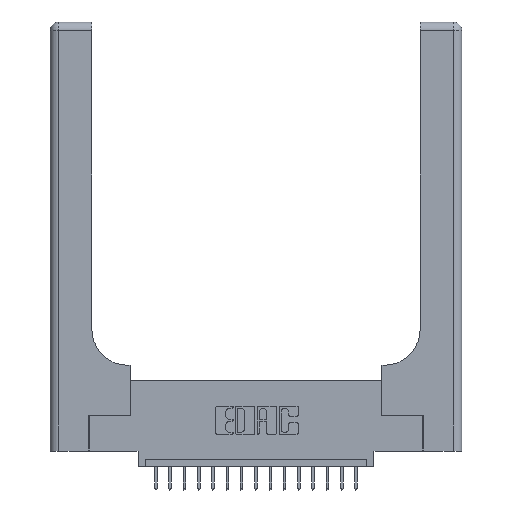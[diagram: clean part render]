
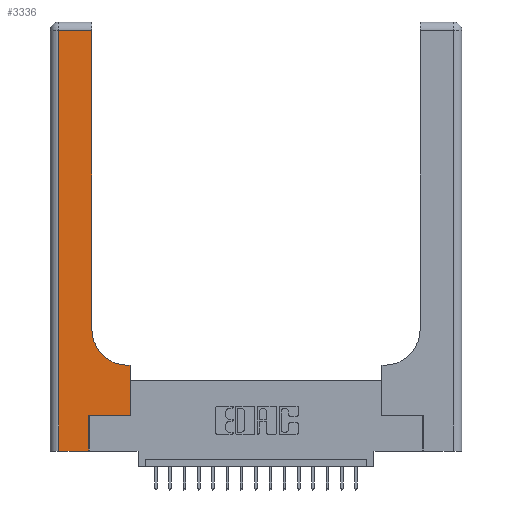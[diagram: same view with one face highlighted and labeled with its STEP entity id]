
A CAD part, top view. The second image highlights one B-rep face of the part: STEP entity #3336.
In plain terms, the highlighted planar face has unit normal (0, 0, 1).
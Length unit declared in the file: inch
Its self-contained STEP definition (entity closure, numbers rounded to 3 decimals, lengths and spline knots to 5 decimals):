
#299 = CARTESIAN_POINT ( 'NONE',  ( 0.5585, 0.6, 0.37 ) ) ;
#445 = DIRECTION ( 'NONE',  ( 1., 0., 0. ) ) ;
#703 = DIRECTION ( 'NONE',  ( 0., 1., 0. ) ) ;
#721 = LINE ( 'NONE', #16272, #4425 ) ;
#781 = ORIENTED_EDGE ( 'NONE', *, *, #13419, .T. ) ;
#2010 = CARTESIAN_POINT ( 'NONE',  ( 0.269, 0., 0.37 ) ) ;
#2020 = ORIENTED_EDGE ( 'NONE', *, *, #5002, .T. ) ;
#2302 = VERTEX_POINT ( 'NONE', #16727 ) ;
#2441 = CIRCLE ( 'NONE', #20282, 0.25 ) ;
#2905 = FACE_OUTER_BOUND ( 'NONE', #6049, .T. ) ;
#2906 = CARTESIAN_POINT ( 'NONE',  ( 0.2915, 0.6, 0.37 ) ) ;
#3103 = VECTOR ( 'NONE', #10601, 39.37008 ) ;
#3206 = VECTOR ( 'NONE', #17125, 39.37008 ) ;
#3258 = CARTESIAN_POINT ( 'NONE',  ( 0.06, 0., 0.37 ) ) ;
#3336 = ADVANCED_FACE ( 'NONE', ( #2905 ), #9201, .F. ) ;
#4198 = VERTEX_POINT ( 'NONE', #6882 ) ;
#4246 = LINE ( 'NONE', #16491, #17465 ) ;
#4425 = VECTOR ( 'NONE', #445, 39.37008 ) ;
#4515 = VECTOR ( 'NONE', #7866, 39.37008 ) ;
#4678 = AXIS2_PLACEMENT_3D ( 'NONE', #18468, #6034, #19993 ) ;
#4734 = VERTEX_POINT ( 'NONE', #14082 ) ;
#5002 = EDGE_CURVE ( 'NONE', #16333, #4198, #7132, .T. ) ;
#5323 = CARTESIAN_POINT ( 'NONE',  ( 0.2915, 2.94, 0.37 ) ) ;
#5723 = VERTEX_POINT ( 'NONE', #299 ) ;
#6034 = DIRECTION ( 'NONE',  ( 0., 0., -1. ) ) ;
#6049 = EDGE_LOOP ( 'NONE', ( #15083, #15637, #16638, #14212, #2020, #15457, #15556, #781, #15235 ) ) ;
#6213 = DIRECTION ( 'NONE',  ( 1., 0., 0. ) ) ;
#6253 = VERTEX_POINT ( 'NONE', #5323 ) ;
#6272 = CARTESIAN_POINT ( 'NONE',  ( 0.2915, 3., 0.37 ) ) ;
#6664 = CARTESIAN_POINT ( 'NONE',  ( 0., 2.94, 0.37 ) ) ;
#6882 = CARTESIAN_POINT ( 'NONE',  ( 0.269, 0.25, 0.37 ) ) ;
#7041 = CARTESIAN_POINT ( 'NONE',  ( 0.06, 2.94, 0.37 ) ) ;
#7132 = LINE ( 'NONE', #14270, #3206 ) ;
#7368 = VERTEX_POINT ( 'NONE', #3258 ) ;
#7866 = DIRECTION ( 'NONE',  ( 0., 1., 0. ) ) ;
#8069 = VECTOR ( 'NONE', #703, 39.37008 ) ;
#8564 = LINE ( 'NONE', #13093, #8069 ) ;
#9201 = PLANE ( 'NONE',  #4678 ) ;
#9466 = EDGE_CURVE ( 'NONE', #18646, #7368, #19944, .T. ) ;
#9497 = DIRECTION ( 'NONE',  ( 0., 0., -1. ) ) ;
#9608 = EDGE_CURVE ( 'NONE', #7368, #16333, #4246, .T. ) ;
#10082 = LINE ( 'NONE', #6664, #18382 ) ;
#10346 = DIRECTION ( 'NONE',  ( 1., 0., 0. ) ) ;
#10476 = CARTESIAN_POINT ( 'NONE',  ( 0.2915, 0.85, 0.37 ) ) ;
#10601 = DIRECTION ( 'NONE',  ( -1., 0., 0. ) ) ;
#12676 = EDGE_CURVE ( 'NONE', #4734, #5723, #8564, .T. ) ;
#13093 = CARTESIAN_POINT ( 'NONE',  ( 0.5585, 0.25, 0.37 ) ) ;
#13419 = EDGE_CURVE ( 'NONE', #5723, #2302, #14632, .T. ) ;
#13652 = VERTEX_POINT ( 'NONE', #10476 ) ;
#14082 = CARTESIAN_POINT ( 'NONE',  ( 0.5585, 0.25, 0.37 ) ) ;
#14212 = ORIENTED_EDGE ( 'NONE', *, *, #9608, .T. ) ;
#14223 = CARTESIAN_POINT ( 'NONE',  ( 0.5415, 0.85, 0.37 ) ) ;
#14270 = CARTESIAN_POINT ( 'NONE',  ( 0.269, 0., 0.37 ) ) ;
#14632 = LINE ( 'NONE', #2906, #3103 ) ;
#15083 = ORIENTED_EDGE ( 'NONE', *, *, #15085, .T. ) ;
#15085 = EDGE_CURVE ( 'NONE', #13652, #6253, #16023, .T. ) ;
#15235 = ORIENTED_EDGE ( 'NONE', *, *, #17080, .T. ) ;
#15457 = ORIENTED_EDGE ( 'NONE', *, *, #18511, .T. ) ;
#15556 = ORIENTED_EDGE ( 'NONE', *, *, #12676, .T. ) ;
#15637 = ORIENTED_EDGE ( 'NONE', *, *, #16813, .T. ) ;
#16023 = LINE ( 'NONE', #6272, #4515 ) ;
#16272 = CARTESIAN_POINT ( 'NONE',  ( 0.269, 0.25, 0.37 ) ) ;
#16333 = VERTEX_POINT ( 'NONE', #2010 ) ;
#16491 = CARTESIAN_POINT ( 'NONE',  ( 0., 0., 0.37 ) ) ;
#16638 = ORIENTED_EDGE ( 'NONE', *, *, #9466, .T. ) ;
#16727 = CARTESIAN_POINT ( 'NONE',  ( 0.5415, 0.6, 0.37 ) ) ;
#16813 = EDGE_CURVE ( 'NONE', #6253, #18646, #10082, .T. ) ;
#17009 = CARTESIAN_POINT ( 'NONE',  ( 0.06, 3., 0.37 ) ) ;
#17080 = EDGE_CURVE ( 'NONE', #2302, #13652, #2441, .T. ) ;
#17125 = DIRECTION ( 'NONE',  ( 0., 1., 0. ) ) ;
#17465 = VECTOR ( 'NONE', #10346, 39.37008 ) ;
#17603 = DIRECTION ( 'NONE',  ( -1., 0., 0. ) ) ;
#18371 = DIRECTION ( 'NONE',  ( 0., -1., 0. ) ) ;
#18382 = VECTOR ( 'NONE', #17603, 39.37008 ) ;
#18460 = VECTOR ( 'NONE', #18371, 39.37008 ) ;
#18468 = CARTESIAN_POINT ( 'NONE',  ( 0., 3., 0.37 ) ) ;
#18511 = EDGE_CURVE ( 'NONE', #4198, #4734, #721, .T. ) ;
#18646 = VERTEX_POINT ( 'NONE', #7041 ) ;
#19944 = LINE ( 'NONE', #17009, #18460 ) ;
#19993 = DIRECTION ( 'NONE',  ( -1., 0., 0. ) ) ;
#20282 = AXIS2_PLACEMENT_3D ( 'NONE', #14223, #9497, #6213 ) ;
